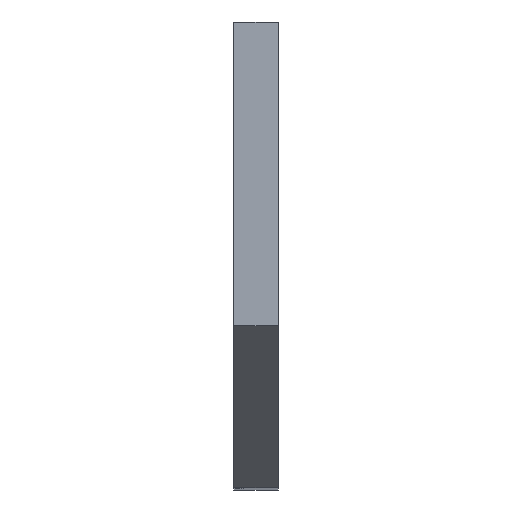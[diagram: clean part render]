
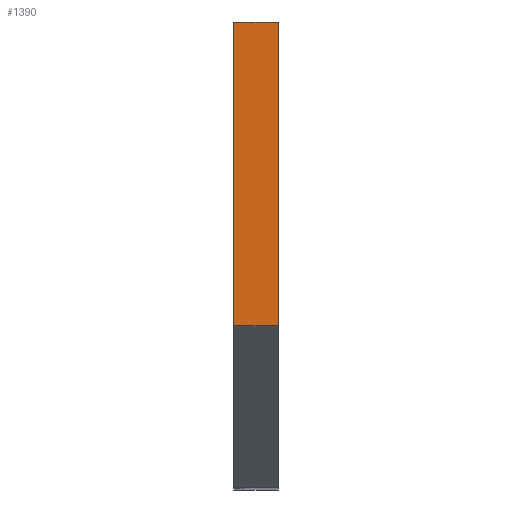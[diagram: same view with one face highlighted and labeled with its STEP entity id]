
A CAD part, top view. The second image highlights one B-rep face of the part: STEP entity #1390.
In plain terms, the highlighted planar face has unit normal (0, 0, 1).
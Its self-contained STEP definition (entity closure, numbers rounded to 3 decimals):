
#46 = CARTESIAN_POINT ( 'NONE',  ( -3.175, 11.608, 0. ) ) ;
#60 = VECTOR ( 'NONE', #701, 1000. ) ;
#80 = VERTEX_POINT ( 'NONE', #927 ) ;
#171 = VERTEX_POINT ( 'NONE', #1545 ) ;
#181 = EDGE_CURVE ( 'NONE', #171, #1163, #547, .T. ) ;
#354 = VECTOR ( 'NONE', #992, 1000. ) ;
#384 = EDGE_CURVE ( 'NONE', #1163, #80, #1690, .T. ) ;
#440 = LINE ( 'NONE', #1691, #354 ) ;
#514 = EDGE_CURVE ( 'NONE', #1592, #80, #440, .T. ) ;
#547 = LINE ( 'NONE', #704, #1255 ) ;
#564 = CARTESIAN_POINT ( 'NONE',  ( -3.175, 33.426, 0. ) ) ;
#598 = ORIENTED_EDGE ( 'NONE', *, *, #384, .T. ) ;
#605 = CARTESIAN_POINT ( 'NONE',  ( -3.175, 11.608, 0. ) ) ;
#684 = ORIENTED_EDGE ( 'NONE', *, *, #181, .T. ) ;
#701 = DIRECTION ( 'NONE',  ( 1., 0., 0. ) ) ;
#704 = CARTESIAN_POINT ( 'NONE',  ( -3.175, 0., 0. ) ) ;
#790 = PLANE ( 'NONE',  #844 ) ;
#797 = CARTESIAN_POINT ( 'NONE',  ( -3.175, 0., 0. ) ) ;
#844 = AXIS2_PLACEMENT_3D ( 'NONE', #797, #1771, #937 ) ;
#848 = DIRECTION ( 'NONE',  ( 0., -1., 0. ) ) ;
#869 = EDGE_LOOP ( 'NONE', ( #1598, #1198, #684, #598 ) ) ;
#927 = CARTESIAN_POINT ( 'NONE',  ( 0., 11.608, 0. ) ) ;
#937 = DIRECTION ( 'NONE',  ( 0., -1., 0. ) ) ;
#992 = DIRECTION ( 'NONE',  ( 0., -1., 0. ) ) ;
#1034 = DIRECTION ( 'NONE',  ( 1., 0., 0. ) ) ;
#1163 = VERTEX_POINT ( 'NONE', #46 ) ;
#1178 = LINE ( 'NONE', #564, #60 ) ;
#1198 = ORIENTED_EDGE ( 'NONE', *, *, #1646, .F. ) ;
#1206 = FACE_OUTER_BOUND ( 'NONE', #869, .T. ) ;
#1255 = VECTOR ( 'NONE', #848, 1000. ) ;
#1264 = CARTESIAN_POINT ( 'NONE',  ( 0., 33.426, 0. ) ) ;
#1320 = VECTOR ( 'NONE', #1034, 1000. ) ;
#1390 = ADVANCED_FACE ( 'NONE', ( #1206 ), #790, .T. ) ;
#1545 = CARTESIAN_POINT ( 'NONE',  ( -3.175, 33.426, 0. ) ) ;
#1592 = VERTEX_POINT ( 'NONE', #1264 ) ;
#1598 = ORIENTED_EDGE ( 'NONE', *, *, #514, .F. ) ;
#1646 = EDGE_CURVE ( 'NONE', #171, #1592, #1178, .T. ) ;
#1690 = LINE ( 'NONE', #605, #1320 ) ;
#1691 = CARTESIAN_POINT ( 'NONE',  ( 0., 0., 0. ) ) ;
#1771 = DIRECTION ( 'NONE',  ( 0., 0., 1. ) ) ;
